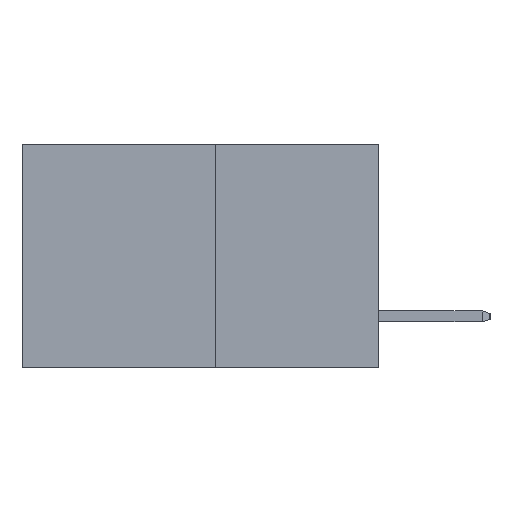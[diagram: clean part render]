
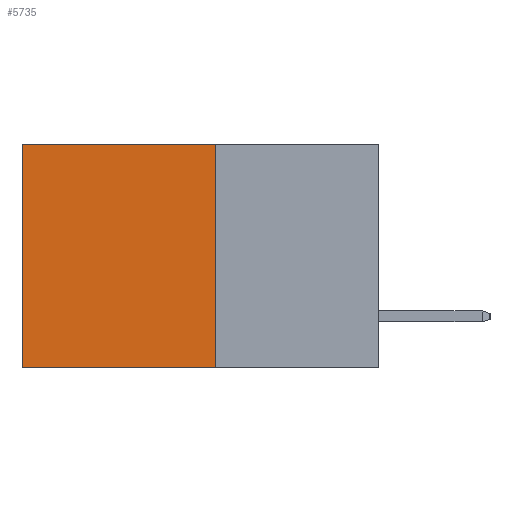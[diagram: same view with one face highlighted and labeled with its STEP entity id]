
A CAD part, left-side view. The second image highlights one B-rep face of the part: STEP entity #5735.
In plain terms, the highlighted planar face has unit normal (-1, 0, 0).
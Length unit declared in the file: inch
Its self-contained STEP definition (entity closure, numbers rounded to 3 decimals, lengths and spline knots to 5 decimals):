
#591 = DIRECTION ( 'NONE',  ( 1., 0., 0. ) ) ;
#594 = PLANE ( 'NONE',  #6919 ) ;
#698 = CARTESIAN_POINT ( 'NONE',  ( 0.277, 0.27, 0. ) ) ;
#708 = DIRECTION ( 'NONE',  ( 0., 0., -1. ) ) ;
#949 = CARTESIAN_POINT ( 'NONE',  ( 0.277, 0.59, -0.37 ) ) ;
#974 = VERTEX_POINT ( 'NONE', #698 ) ;
#1646 = VECTOR ( 'NONE', #2514, 39.37008 ) ;
#2247 = LINE ( 'NONE', #2471, #1646 ) ;
#2471 = CARTESIAN_POINT ( 'NONE',  ( 0.277, 0.27, -0.37 ) ) ;
#2514 = DIRECTION ( 'NONE',  ( 0., 1., 0. ) ) ;
#2761 = ORIENTED_EDGE ( 'NONE', *, *, #10012, .F. ) ;
#2797 = VERTEX_POINT ( 'NONE', #949 ) ;
#3051 = LINE ( 'NONE', #3730, #5085 ) ;
#3212 = CARTESIAN_POINT ( 'NONE',  ( 0.277, 0.27, -0.37 ) ) ;
#3650 = VECTOR ( 'NONE', #10507, 39.37008 ) ;
#3658 = DIRECTION ( 'NONE',  ( 0., 1., 0. ) ) ;
#3730 = CARTESIAN_POINT ( 'NONE',  ( 0.277, 0.27, 0. ) ) ;
#4549 = DIRECTION ( 'NONE',  ( 0., 0., -1. ) ) ;
#5085 = VECTOR ( 'NONE', #3658, 39.37008 ) ;
#5608 = ORIENTED_EDGE ( 'NONE', *, *, #7847, .T. ) ;
#5622 = ORIENTED_EDGE ( 'NONE', *, *, #10219, .T. ) ;
#5735 = ADVANCED_FACE ( 'NONE', ( #8741 ), #594, .F. ) ;
#5821 = VECTOR ( 'NONE', #708, 39.37008 ) ;
#6876 = CARTESIAN_POINT ( 'NONE',  ( 0.277, 0.27, -0.37 ) ) ;
#6919 = AXIS2_PLACEMENT_3D ( 'NONE', #6876, #591, #4549 ) ;
#7847 = EDGE_CURVE ( 'NONE', #974, #10717, #3051, .T. ) ;
#7896 = VERTEX_POINT ( 'NONE', #3212 ) ;
#7969 = EDGE_CURVE ( 'NONE', #7896, #2797, #2247, .T. ) ;
#8217 = LINE ( 'NONE', #9696, #3650 ) ;
#8357 = LINE ( 'NONE', #9440, #5821 ) ;
#8681 = CARTESIAN_POINT ( 'NONE',  ( 0.277, 0.59, 0. ) ) ;
#8741 = FACE_OUTER_BOUND ( 'NONE', #10867, .T. ) ;
#9357 = ORIENTED_EDGE ( 'NONE', *, *, #7969, .F. ) ;
#9440 = CARTESIAN_POINT ( 'NONE',  ( 0.277, 0.27, -0.37 ) ) ;
#9696 = CARTESIAN_POINT ( 'NONE',  ( 0.277, 0.59, -0.37 ) ) ;
#10012 = EDGE_CURVE ( 'NONE', #974, #7896, #8357, .T. ) ;
#10219 = EDGE_CURVE ( 'NONE', #10717, #2797, #8217, .T. ) ;
#10507 = DIRECTION ( 'NONE',  ( 0., 0., -1. ) ) ;
#10717 = VERTEX_POINT ( 'NONE', #8681 ) ;
#10867 = EDGE_LOOP ( 'NONE', ( #5622, #9357, #2761, #5608 ) ) ;
